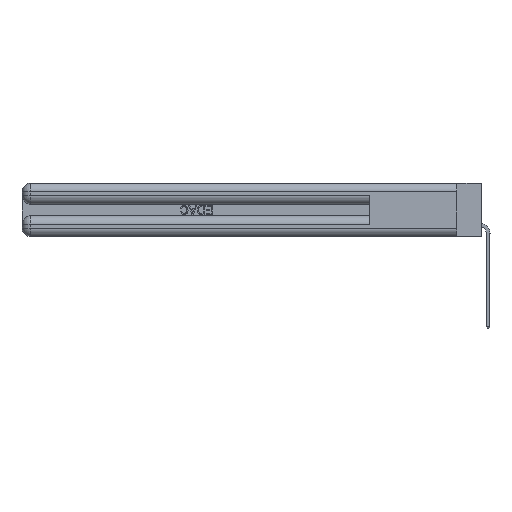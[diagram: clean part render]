
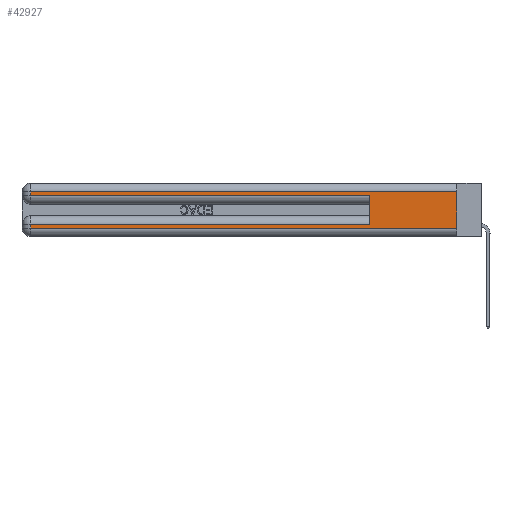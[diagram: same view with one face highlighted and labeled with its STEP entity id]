
A CAD part, left-side view. The second image highlights one B-rep face of the part: STEP entity #42927.
In plain terms, the highlighted planar face has unit normal (-1, 0, 0).
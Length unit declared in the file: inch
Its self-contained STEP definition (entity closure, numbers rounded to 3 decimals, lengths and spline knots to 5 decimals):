
#1074 = CARTESIAN_POINT ( 'NONE',  ( 0., 2.94, 0.285 ) ) ;
#2211 = AXIS2_PLACEMENT_3D ( 'NONE', #15252, #44595, #32076 ) ;
#2753 = ORIENTED_EDGE ( 'NONE', *, *, #6655, .T. ) ;
#3290 = LINE ( 'NONE', #24775, #47989 ) ;
#4694 = LINE ( 'NONE', #49229, #21575 ) ;
#5320 = ORIENTED_EDGE ( 'NONE', *, *, #43462, .F. ) ;
#5437 = VERTEX_POINT ( 'NONE', #36824 ) ;
#6655 = EDGE_CURVE ( 'NONE', #46988, #23630, #42849, .T. ) ;
#6877 = PLANE ( 'NONE',  #2211 ) ;
#7269 = VERTEX_POINT ( 'NONE', #21342 ) ;
#7502 = VERTEX_POINT ( 'NONE', #24318 ) ;
#7937 = DIRECTION ( 'NONE',  ( 0., -1., 0. ) ) ;
#8587 = DIRECTION ( 'NONE',  ( 0., 0., -1. ) ) ;
#9326 = VECTOR ( 'NONE', #28868, 39.37008 ) ;
#9467 = ORIENTED_EDGE ( 'NONE', *, *, #45753, .T. ) ;
#10098 = EDGE_CURVE ( 'NONE', #44431, #5437, #24162, .T. ) ;
#12044 = CARTESIAN_POINT ( 'NONE',  ( 0., 2.94, 0.37 ) ) ;
#13030 = VECTOR ( 'NONE', #36785, 39.37008 ) ;
#13083 = CARTESIAN_POINT ( 'NONE',  ( 0., 0., 0.285 ) ) ;
#15062 = VECTOR ( 'NONE', #33295, 39.37008 ) ;
#15252 = CARTESIAN_POINT ( 'NONE',  ( 0., 0., 0.37 ) ) ;
#15981 = LINE ( 'NONE', #12044, #9326 ) ;
#17107 = FACE_OUTER_BOUND ( 'NONE', #53634, .T. ) ;
#18450 = DIRECTION ( 'NONE',  ( 0., 1., 0. ) ) ;
#19557 = CARTESIAN_POINT ( 'NONE',  ( 0., 0.6, 0.145 ) ) ;
#21342 = CARTESIAN_POINT ( 'NONE',  ( 0., 0.6, 0.085 ) ) ;
#21575 = VECTOR ( 'NONE', #7937, 39.37008 ) ;
#21817 = CARTESIAN_POINT ( 'NONE',  ( 0., 0., 0.37 ) ) ;
#22624 = CARTESIAN_POINT ( 'NONE',  ( 0., 0., 0.085 ) ) ;
#23630 = VERTEX_POINT ( 'NONE', #45413 ) ;
#24162 = LINE ( 'NONE', #41089, #13030 ) ;
#24318 = CARTESIAN_POINT ( 'NONE',  ( 0., 2.94, 0.085 ) ) ;
#24516 = VERTEX_POINT ( 'NONE', #31572 ) ;
#24775 = CARTESIAN_POINT ( 'NONE',  ( 0., 2.94, 0.37 ) ) ;
#24827 = EDGE_CURVE ( 'NONE', #7269, #7502, #33105, .T. ) ;
#28097 = ORIENTED_EDGE ( 'NONE', *, *, #10098, .T. ) ;
#28103 = VERTEX_POINT ( 'NONE', #46084 ) ;
#28868 = DIRECTION ( 'NONE',  ( 0., 0., -1. ) ) ;
#31214 = ORIENTED_EDGE ( 'NONE', *, *, #43365, .T. ) ;
#31572 = CARTESIAN_POINT ( 'NONE',  ( 0., 0., 0.06 ) ) ;
#32076 = DIRECTION ( 'NONE',  ( 0., 0., -1. ) ) ;
#33105 = LINE ( 'NONE', #22624, #52516 ) ;
#33191 = ORIENTED_EDGE ( 'NONE', *, *, #24827, .T. ) ;
#33295 = DIRECTION ( 'NONE',  ( 0., -1., 0. ) ) ;
#33406 = DIRECTION ( 'NONE',  ( 0., 0., 1. ) ) ;
#35871 = LINE ( 'NONE', #21817, #46757 ) ;
#36785 = DIRECTION ( 'NONE',  ( 0., 1., 0. ) ) ;
#36824 = CARTESIAN_POINT ( 'NONE',  ( 0., 2.94, 0.31 ) ) ;
#39284 = EDGE_CURVE ( 'NONE', #7269, #23630, #39383, .T. ) ;
#39383 = LINE ( 'NONE', #19557, #47802 ) ;
#40671 = EDGE_CURVE ( 'NONE', #5437, #46988, #15981, .T. ) ;
#40997 = ORIENTED_EDGE ( 'NONE', *, *, #39284, .F. ) ;
#41089 = CARTESIAN_POINT ( 'NONE',  ( 0., 0., 0.31 ) ) ;
#42849 = LINE ( 'NONE', #13083, #15062 ) ;
#42927 = ADVANCED_FACE ( 'NONE', ( #17107 ), #6877, .F. ) ;
#43365 = EDGE_CURVE ( 'NONE', #28103, #24516, #4694, .T. ) ;
#43462 = EDGE_CURVE ( 'NONE', #44431, #24516, #35871, .T. ) ;
#44431 = VERTEX_POINT ( 'NONE', #52536 ) ;
#44595 = DIRECTION ( 'NONE',  ( 1., 0., 0. ) ) ;
#45413 = CARTESIAN_POINT ( 'NONE',  ( 0., 0.6, 0.285 ) ) ;
#45753 = EDGE_CURVE ( 'NONE', #7502, #28103, #3290, .T. ) ;
#46084 = CARTESIAN_POINT ( 'NONE',  ( 0., 2.94, 0.06 ) ) ;
#46757 = VECTOR ( 'NONE', #8587, 39.37008 ) ;
#46988 = VERTEX_POINT ( 'NONE', #1074 ) ;
#47802 = VECTOR ( 'NONE', #33406, 39.37008 ) ;
#47989 = VECTOR ( 'NONE', #50194, 39.37008 ) ;
#49229 = CARTESIAN_POINT ( 'NONE',  ( 0., 0., 0.06 ) ) ;
#49611 = ORIENTED_EDGE ( 'NONE', *, *, #40671, .T. ) ;
#50194 = DIRECTION ( 'NONE',  ( 0., 0., -1. ) ) ;
#52516 = VECTOR ( 'NONE', #18450, 39.37008 ) ;
#52536 = CARTESIAN_POINT ( 'NONE',  ( 0., 0., 0.31 ) ) ;
#53634 = EDGE_LOOP ( 'NONE', ( #5320, #28097, #49611, #2753, #40997, #33191, #9467, #31214 ) ) ;
